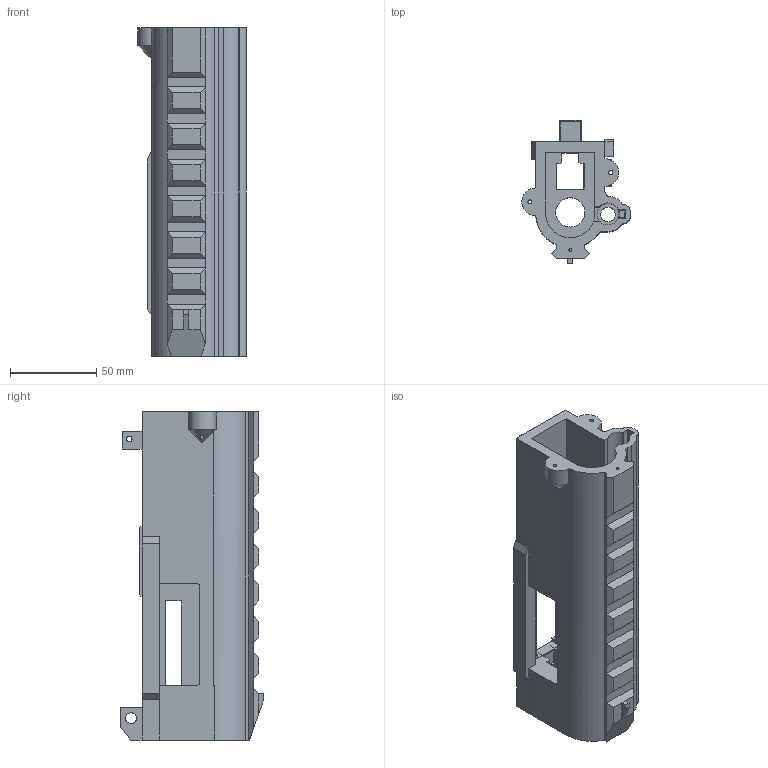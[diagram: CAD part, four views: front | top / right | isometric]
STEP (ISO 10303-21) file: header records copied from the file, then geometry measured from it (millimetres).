
FILE_DESCRIPTION (( 'STEP AP203' ), '1' );
FILE_NAME ('WTF-9H_upper_receiver.STEP', '2020-06-09T21:46:44', ( '' ), ( '' ), 'SwSTEP 2.0', 'SolidWorks 2016', '' );
FILE_SCHEMA (( 'CONFIG_CONTROL_DESIGN' ));
Length unit declared in the file: millimetre
Products named in the file (1): WTF-9H_upper_receiver
Bounding box: 62.82 x 83.5 x 190.38 mm (x, y, z)
Volume: 231160.3 mm3; surface area: 81651.3 mm2
Topology: 1 solids, 1 shells, 290 faces, 811 edges, 522 vertices
Faces by surface type: plane 221, cylinder 53, cone 7, torus 5, bspline 2, sphere 2
Full cylindrical faces by diameter (mm): 1.7 x1, 2.2 x1, 2.4 x5, 2.6 x2, 3.175 x1, 6.375 x1, 8.4 x1, 12.8 x1, 17 x1
Entity records: 9386 total; most frequent: CARTESIAN_POINT 1861, ORIENTED_EDGE 1576, DIRECTION 1459, EDGE_CURVE 788, VECTOR 655, LINE 655, VERTEX_POINT 519, AXIS2_PLACEMENT_3D 402
